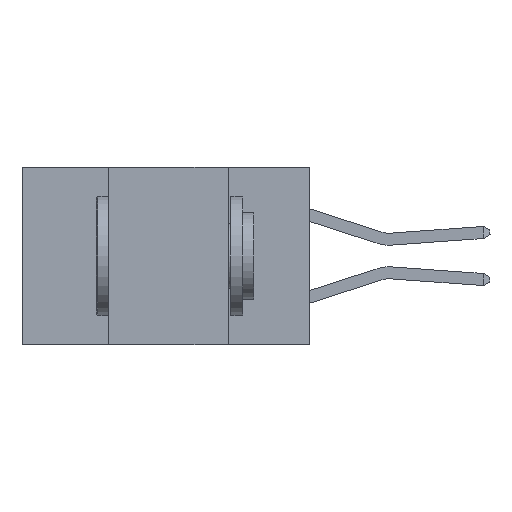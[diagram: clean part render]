
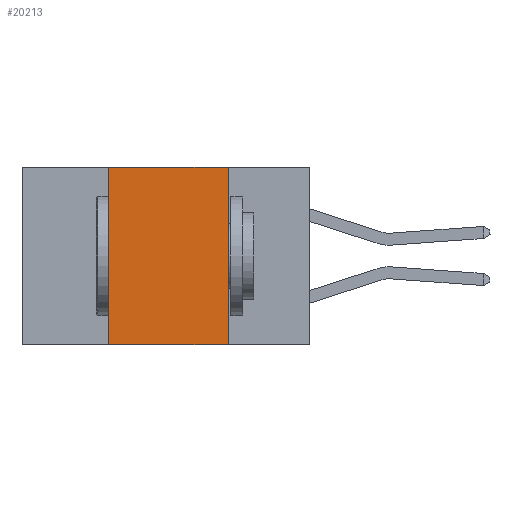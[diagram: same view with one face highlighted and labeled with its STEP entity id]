
A CAD part, left-side view. The second image highlights one B-rep face of the part: STEP entity #20213.
In plain terms, the highlighted planar face has unit normal (-1, 0, 0).
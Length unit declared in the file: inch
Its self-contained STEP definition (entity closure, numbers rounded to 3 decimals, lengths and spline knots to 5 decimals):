
#536 = EDGE_CURVE ( 'NONE', #13437, #6729, #13023, .T. ) ;
#586 = CARTESIAN_POINT ( 'NONE',  ( 0., 0.6, 0. ) ) ;
#811 = ORIENTED_EDGE ( 'NONE', *, *, #2724, .F. ) ;
#905 = LINE ( 'NONE', #18802, #4719 ) ;
#1325 = CARTESIAN_POINT ( 'NONE',  ( 0., 0.6, -0.37 ) ) ;
#1829 = ORIENTED_EDGE ( 'NONE', *, *, #11848, .F. ) ;
#2665 = CARTESIAN_POINT ( 'NONE',  ( 0., 0.17, 0. ) ) ;
#2724 = EDGE_CURVE ( 'NONE', #18054, #6729, #15881, .T. ) ;
#3039 = VERTEX_POINT ( 'NONE', #3438 ) ;
#3160 = CARTESIAN_POINT ( 'NONE',  ( 0., 0.17, -0.37 ) ) ;
#3438 = CARTESIAN_POINT ( 'NONE',  ( 0., 0.42, 0. ) ) ;
#3527 = FACE_OUTER_BOUND ( 'NONE', #17903, .T. ) ;
#3936 = DIRECTION ( 'NONE',  ( 0., 0., -1. ) ) ;
#4719 = VECTOR ( 'NONE', #9318, 39.37008 ) ;
#6729 = VERTEX_POINT ( 'NONE', #3160 ) ;
#7316 = VECTOR ( 'NONE', #7783, 39.37008 ) ;
#7783 = DIRECTION ( 'NONE',  ( 0., 0., 1. ) ) ;
#7892 = VECTOR ( 'NONE', #3936, 39.37008 ) ;
#9318 = DIRECTION ( 'NONE',  ( 0., -1., 0. ) ) ;
#9544 = CARTESIAN_POINT ( 'NONE',  ( 0., 0.17, 0. ) ) ;
#10067 = DIRECTION ( 'NONE',  ( 0., 0., -1. ) ) ;
#10309 = ORIENTED_EDGE ( 'NONE', *, *, #10612, .F. ) ;
#10612 = EDGE_CURVE ( 'NONE', #3039, #18054, #905, .T. ) ;
#11848 = EDGE_CURVE ( 'NONE', #13437, #3039, #24117, .T. ) ;
#12188 = PLANE ( 'NONE',  #20989 ) ;
#13023 = LINE ( 'NONE', #1325, #18621 ) ;
#13437 = VERTEX_POINT ( 'NONE', #21293 ) ;
#15881 = LINE ( 'NONE', #9544, #7892 ) ;
#17083 = CARTESIAN_POINT ( 'NONE',  ( 0., 0.42, 0. ) ) ;
#17903 = EDGE_LOOP ( 'NONE', ( #811, #10309, #1829, #24130 ) ) ;
#18054 = VERTEX_POINT ( 'NONE', #2665 ) ;
#18142 = DIRECTION ( 'NONE',  ( 0., -1., 0. ) ) ;
#18621 = VECTOR ( 'NONE', #18142, 39.37008 ) ;
#18802 = CARTESIAN_POINT ( 'NONE',  ( 0., 0.6, 0. ) ) ;
#20213 = ADVANCED_FACE ( 'NONE', ( #3527 ), #12188, .F. ) ;
#20989 = AXIS2_PLACEMENT_3D ( 'NONE', #586, #21428, #10067 ) ;
#21293 = CARTESIAN_POINT ( 'NONE',  ( 0., 0.42, -0.37 ) ) ;
#21428 = DIRECTION ( 'NONE',  ( 1., 0., 0. ) ) ;
#24117 = LINE ( 'NONE', #17083, #7316 ) ;
#24130 = ORIENTED_EDGE ( 'NONE', *, *, #536, .T. ) ;
